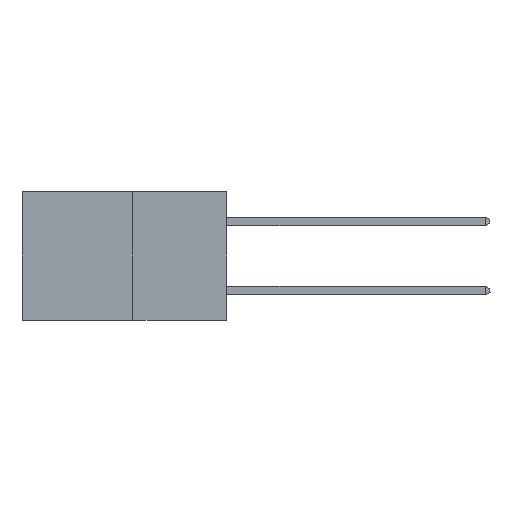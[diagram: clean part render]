
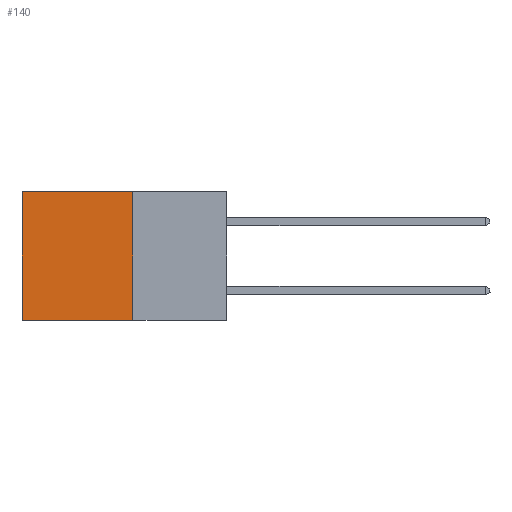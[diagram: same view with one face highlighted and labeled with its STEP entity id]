
A CAD part, left-side view. The second image highlights one B-rep face of the part: STEP entity #140.
In plain terms, the highlighted planar face has unit normal (-1, 0, 0).
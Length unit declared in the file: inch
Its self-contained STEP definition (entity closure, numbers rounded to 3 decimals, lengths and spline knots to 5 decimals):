
#57 = ORIENTED_EDGE ( 'NONE', *, *, #5715, .T. ) ;
#140 = ADVANCED_FACE ( 'NONE', ( #4942 ), #7988, .F. ) ;
#218 = LINE ( 'NONE', #9603, #2066 ) ;
#800 = DIRECTION ( 'NONE',  ( 0., 1., 0. ) ) ;
#1637 = CARTESIAN_POINT ( 'NONE',  ( 0.277, 0.27, -0.37 ) ) ;
#1657 = DIRECTION ( 'NONE',  ( 0., 0., -1. ) ) ;
#1802 = VERTEX_POINT ( 'NONE', #4783 ) ;
#2066 = VECTOR ( 'NONE', #8367, 39.37008 ) ;
#2222 = LINE ( 'NONE', #2502, #6172 ) ;
#2502 = CARTESIAN_POINT ( 'NONE',  ( 0.277, 0.27, -0.37 ) ) ;
#2536 = DIRECTION ( 'NONE',  ( 0., 0., -1. ) ) ;
#2668 = VERTEX_POINT ( 'NONE', #3031 ) ;
#2720 = VERTEX_POINT ( 'NONE', #9337 ) ;
#2955 = VECTOR ( 'NONE', #2983, 39.37008 ) ;
#2983 = DIRECTION ( 'NONE',  ( 0., 1., 0. ) ) ;
#3019 = CARTESIAN_POINT ( 'NONE',  ( 0.277, 0.27, 0. ) ) ;
#3031 = CARTESIAN_POINT ( 'NONE',  ( 0.277, 0.59, -0.37 ) ) ;
#3353 = AXIS2_PLACEMENT_3D ( 'NONE', #8678, #5227, #1657 ) ;
#3507 = LINE ( 'NONE', #1637, #5853 ) ;
#4048 = ORIENTED_EDGE ( 'NONE', *, *, #7150, .T. ) ;
#4783 = CARTESIAN_POINT ( 'NONE',  ( 0.277, 0.59, 0. ) ) ;
#4888 = EDGE_CURVE ( 'NONE', #7774, #2668, #3507, .T. ) ;
#4942 = FACE_OUTER_BOUND ( 'NONE', #9246, .T. ) ;
#5227 = DIRECTION ( 'NONE',  ( 1., 0., 0. ) ) ;
#5715 = EDGE_CURVE ( 'NONE', #2720, #1802, #7130, .T. ) ;
#5768 = EDGE_CURVE ( 'NONE', #2720, #7774, #2222, .T. ) ;
#5853 = VECTOR ( 'NONE', #800, 39.37008 ) ;
#6106 = ORIENTED_EDGE ( 'NONE', *, *, #4888, .F. ) ;
#6172 = VECTOR ( 'NONE', #2536, 39.37008 ) ;
#7130 = LINE ( 'NONE', #3019, #2955 ) ;
#7150 = EDGE_CURVE ( 'NONE', #1802, #2668, #218, .T. ) ;
#7774 = VERTEX_POINT ( 'NONE', #9099 ) ;
#7988 = PLANE ( 'NONE',  #3353 ) ;
#8122 = ORIENTED_EDGE ( 'NONE', *, *, #5768, .F. ) ;
#8367 = DIRECTION ( 'NONE',  ( 0., 0., -1. ) ) ;
#8678 = CARTESIAN_POINT ( 'NONE',  ( 0.277, 0.27, -0.37 ) ) ;
#9099 = CARTESIAN_POINT ( 'NONE',  ( 0.277, 0.27, -0.37 ) ) ;
#9246 = EDGE_LOOP ( 'NONE', ( #4048, #6106, #8122, #57 ) ) ;
#9337 = CARTESIAN_POINT ( 'NONE',  ( 0.277, 0.27, 0. ) ) ;
#9603 = CARTESIAN_POINT ( 'NONE',  ( 0.277, 0.59, -0.37 ) ) ;
